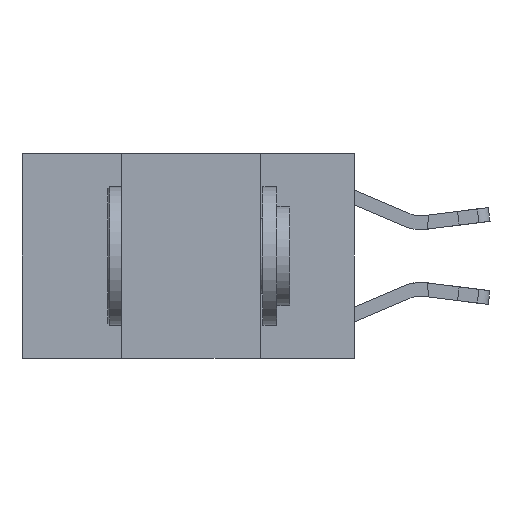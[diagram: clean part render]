
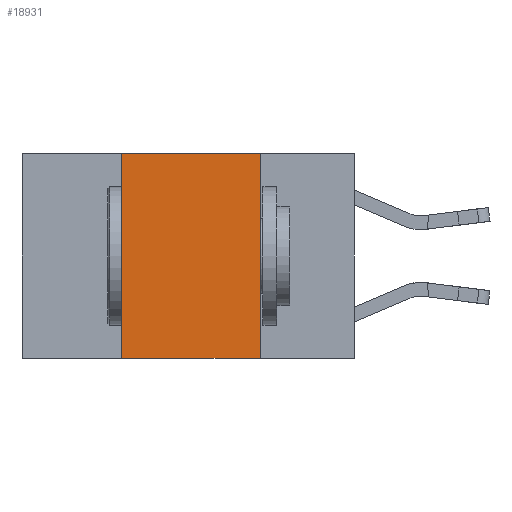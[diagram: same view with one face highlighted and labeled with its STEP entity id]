
A CAD part, left-side view. The second image highlights one B-rep face of the part: STEP entity #18931.
In plain terms, the highlighted planar face has unit normal (-1, 0, 0).
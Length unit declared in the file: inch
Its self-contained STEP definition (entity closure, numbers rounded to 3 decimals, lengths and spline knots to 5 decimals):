
#635 = PLANE ( 'NONE',  #12482 ) ;
#1980 = LINE ( 'NONE', #5863, #25248 ) ;
#2931 = EDGE_CURVE ( 'NONE', #25555, #4390, #11826, .T. ) ;
#3533 = CARTESIAN_POINT ( 'NONE',  ( 0., 0.42, 0. ) ) ;
#3651 = CARTESIAN_POINT ( 'NONE',  ( 0., 0.17, -0.37 ) ) ;
#3742 = EDGE_CURVE ( 'NONE', #13851, #8735, #5274, .T. ) ;
#4192 = ORIENTED_EDGE ( 'NONE', *, *, #28437, .T. ) ;
#4390 = VERTEX_POINT ( 'NONE', #3651 ) ;
#5231 = DIRECTION ( 'NONE',  ( 1., 0., 0. ) ) ;
#5274 = LINE ( 'NONE', #18218, #21856 ) ;
#5863 = CARTESIAN_POINT ( 'NONE',  ( 0., 0.6, 0. ) ) ;
#7059 = EDGE_CURVE ( 'NONE', #8735, #25555, #1980, .T. ) ;
#7535 = DIRECTION ( 'NONE',  ( 0., 0., -1. ) ) ;
#8551 = ORIENTED_EDGE ( 'NONE', *, *, #7059, .F. ) ;
#8735 = VERTEX_POINT ( 'NONE', #3533 ) ;
#9605 = CARTESIAN_POINT ( 'NONE',  ( 0., 0.42, -0.37 ) ) ;
#11826 = LINE ( 'NONE', #20596, #15853 ) ;
#12042 = CARTESIAN_POINT ( 'NONE',  ( 0., 0.6, -0.37 ) ) ;
#12482 = AXIS2_PLACEMENT_3D ( 'NONE', #26996, #5231, #7535 ) ;
#13244 = ORIENTED_EDGE ( 'NONE', *, *, #2931, .F. ) ;
#13851 = VERTEX_POINT ( 'NONE', #9605 ) ;
#15853 = VECTOR ( 'NONE', #27388, 39.37008 ) ;
#17303 = VECTOR ( 'NONE', #23426, 39.37008 ) ;
#17344 = CARTESIAN_POINT ( 'NONE',  ( 0., 0.17, 0. ) ) ;
#18218 = CARTESIAN_POINT ( 'NONE',  ( 0., 0.42, 0. ) ) ;
#18931 = ADVANCED_FACE ( 'NONE', ( #20346 ), #635, .F. ) ;
#19235 = DIRECTION ( 'NONE',  ( 0., -1., 0. ) ) ;
#20346 = FACE_OUTER_BOUND ( 'NONE', #27285, .T. ) ;
#20596 = CARTESIAN_POINT ( 'NONE',  ( 0., 0.17, 0. ) ) ;
#21856 = VECTOR ( 'NONE', #22842, 39.37008 ) ;
#22842 = DIRECTION ( 'NONE',  ( 0., 0., 1. ) ) ;
#23275 = LINE ( 'NONE', #12042, #17303 ) ;
#23426 = DIRECTION ( 'NONE',  ( 0., -1., 0. ) ) ;
#25248 = VECTOR ( 'NONE', #19235, 39.37008 ) ;
#25555 = VERTEX_POINT ( 'NONE', #17344 ) ;
#26996 = CARTESIAN_POINT ( 'NONE',  ( 0., 0.6, 0. ) ) ;
#27285 = EDGE_LOOP ( 'NONE', ( #13244, #8551, #27555, #4192 ) ) ;
#27388 = DIRECTION ( 'NONE',  ( 0., 0., -1. ) ) ;
#27555 = ORIENTED_EDGE ( 'NONE', *, *, #3742, .F. ) ;
#28437 = EDGE_CURVE ( 'NONE', #13851, #4390, #23275, .T. ) ;
